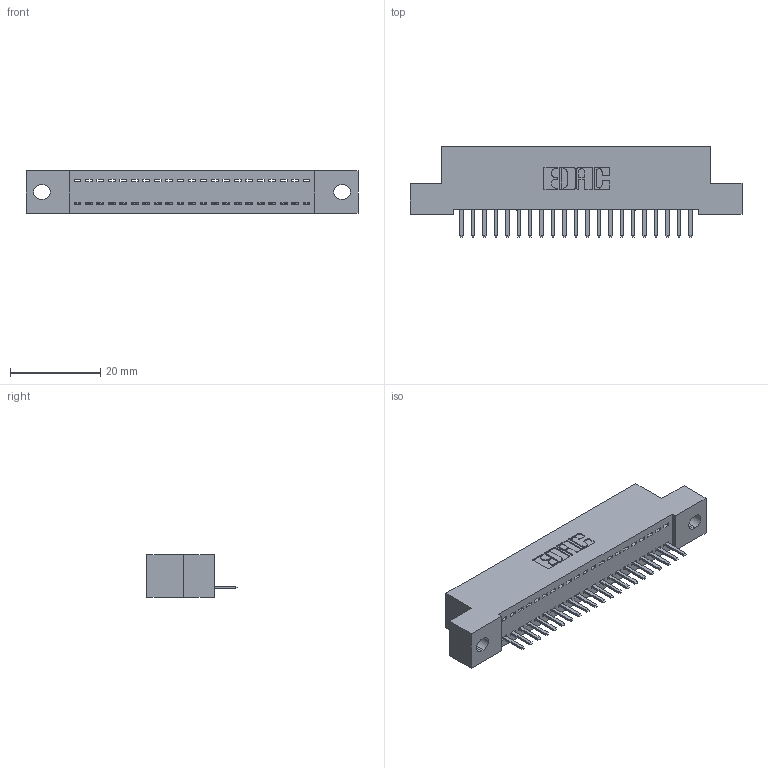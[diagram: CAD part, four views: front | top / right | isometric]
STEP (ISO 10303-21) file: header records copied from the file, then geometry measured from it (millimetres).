
FILE_DESCRIPTION (( 'STEP AP203' ), '1' );
FILE_NAME ('392-021-520-102.STEP', '2019-10-07T05:35:39', ( '' ), ( '' ), 'SwSTEP 2.0', 'SolidWorks 2016', '' );
FILE_SCHEMA (( 'CONFIG_CONTROL_DESIGN' ));
Length unit declared in the file: inch
Products named in the file (3): 342 Part_.128 Slot; 345-292-001_345-293-120; 392-021-520-102
Assembly tree (22 placements, depth 2):
  392-021-520-102
    342 Part_.128 Slot
    345-292-001_345-293-120  x21
Bounding box: 73.66 x 20.02 x 9.4 mm (x, y, z)
Volume: 6268.6 mm3; surface area: 8379.5 mm2
Topology: 22 solids, 22 shells, 1416 faces, 4175 edges, 2726 vertices
Faces by surface type: plane 994, cylinder 422
Entity records: 15671 total; most frequent: CARTESIAN_POINT 2725, ORIENTED_EDGE 2670, DIRECTION 2329, EDGE_CURVE 1335, LINE 1203, VECTOR 1203, VERTEX_POINT 886, AXIS2_PLACEMENT_3D 563
